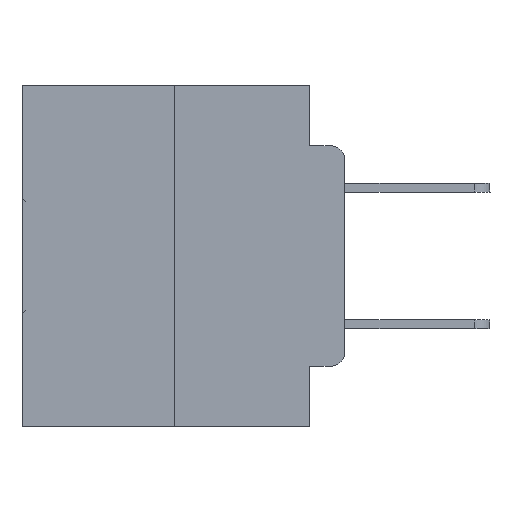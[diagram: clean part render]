
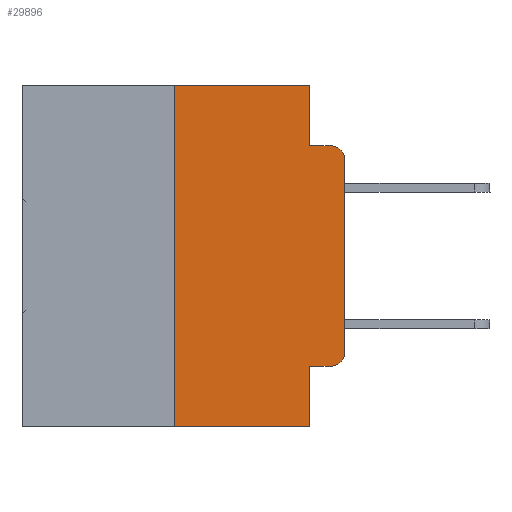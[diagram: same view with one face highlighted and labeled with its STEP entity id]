
A CAD part, left-side view. The second image highlights one B-rep face of the part: STEP entity #29896.
In plain terms, the highlighted planar face has unit normal (-1, 0, 0).
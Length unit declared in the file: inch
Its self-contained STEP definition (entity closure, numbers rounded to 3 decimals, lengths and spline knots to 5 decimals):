
#251 = CARTESIAN_POINT ( 'NONE',  ( 0., 0.051, 0. ) ) ;
#461 = DIRECTION ( 'NONE',  ( 0., -1., 0. ) ) ;
#693 = DIRECTION ( 'NONE',  ( 0., 0., -1. ) ) ;
#1425 = VERTEX_POINT ( 'NONE', #11862 ) ;
#2590 = EDGE_CURVE ( 'NONE', #15403, #14087, #17439, .T. ) ;
#2677 = CARTESIAN_POINT ( 'NONE',  ( 0., 0.02, -0.0885 ) ) ;
#3203 = ORIENTED_EDGE ( 'NONE', *, *, #27578, .F. ) ;
#3482 = DIRECTION ( 'NONE',  ( 0., 0., -1. ) ) ;
#4681 = VECTOR ( 'NONE', #26832, 39.37008 ) ;
#4895 = ORIENTED_EDGE ( 'NONE', *, *, #20392, .T. ) ;
#5065 = VERTEX_POINT ( 'NONE', #13213 ) ;
#5079 = DIRECTION ( 'NONE',  ( -1., 0., 0. ) ) ;
#5665 = VECTOR ( 'NONE', #3482, 39.37008 ) ;
#5751 = CARTESIAN_POINT ( 'NONE',  ( 0., 0.051, -0.0885 ) ) ;
#7278 = EDGE_LOOP ( 'NONE', ( #19356, #32221, #27147, #3203, #12498, #8711, #18273, #20991, #24960, #4895 ) ) ;
#7427 = CARTESIAN_POINT ( 'NONE',  ( 0., 0.051, -0.4115 ) ) ;
#7637 = DIRECTION ( 'NONE',  ( 0., 0., -1. ) ) ;
#8510 = DIRECTION ( 'NONE',  ( 0., -1., 0. ) ) ;
#8711 = ORIENTED_EDGE ( 'NONE', *, *, #25405, .F. ) ;
#9150 = EDGE_CURVE ( 'NONE', #17192, #9315, #14509, .T. ) ;
#9315 = VERTEX_POINT ( 'NONE', #21092 ) ;
#10028 = CARTESIAN_POINT ( 'NONE',  ( 0., 0.02, -0.3915 ) ) ;
#10071 = CARTESIAN_POINT ( 'NONE',  ( 0., 0., 0. ) ) ;
#10776 = EDGE_CURVE ( 'NONE', #25281, #31909, #28466, .T. ) ;
#11602 = DIRECTION ( 'NONE',  ( 0., -1., 0. ) ) ;
#11862 = CARTESIAN_POINT ( 'NONE',  ( 0., 0., -0.3915 ) ) ;
#11918 = AXIS2_PLACEMENT_3D ( 'NONE', #22480, #22384, #7637 ) ;
#12401 = LINE ( 'NONE', #10071, #26482 ) ;
#12488 = PLANE ( 'NONE',  #11918 ) ;
#12498 = ORIENTED_EDGE ( 'NONE', *, *, #10776, .F. ) ;
#12736 = LINE ( 'NONE', #16044, #5665 ) ;
#13051 = CARTESIAN_POINT ( 'NONE',  ( 0., 0.02, -0.1085 ) ) ;
#13213 = CARTESIAN_POINT ( 'NONE',  ( 0., 0.051, -0.5 ) ) ;
#14087 = VERTEX_POINT ( 'NONE', #2677 ) ;
#14341 = CARTESIAN_POINT ( 'NONE',  ( 0., 0.473, 0. ) ) ;
#14509 = LINE ( 'NONE', #7427, #31758 ) ;
#15403 = VERTEX_POINT ( 'NONE', #30290 ) ;
#16044 = CARTESIAN_POINT ( 'NONE',  ( 0., 0.051, 0. ) ) ;
#16433 = CARTESIAN_POINT ( 'NONE',  ( 0., 0.25, 0. ) ) ;
#17080 = CARTESIAN_POINT ( 'NONE',  ( 0., 0.051, 0. ) ) ;
#17192 = VERTEX_POINT ( 'NONE', #25063 ) ;
#17289 = EDGE_CURVE ( 'NONE', #29818, #14087, #26398, .T. ) ;
#17439 = LINE ( 'NONE', #5751, #18234 ) ;
#17487 = DIRECTION ( 'NONE',  ( 0., -1., 0. ) ) ;
#17661 = VERTEX_POINT ( 'NONE', #20322 ) ;
#18234 = VECTOR ( 'NONE', #461, 39.37008 ) ;
#18273 = ORIENTED_EDGE ( 'NONE', *, *, #30205, .T. ) ;
#19356 = ORIENTED_EDGE ( 'NONE', *, *, #21573, .T. ) ;
#20322 = CARTESIAN_POINT ( 'NONE',  ( 0., 0.25, -0.5 ) ) ;
#20392 = EDGE_CURVE ( 'NONE', #9315, #1425, #24549, .T. ) ;
#20574 = VECTOR ( 'NONE', #32305, 39.37008 ) ;
#20762 = DIRECTION ( 'NONE',  ( -1., 0., 0. ) ) ;
#20991 = ORIENTED_EDGE ( 'NONE', *, *, #28213, .F. ) ;
#21092 = CARTESIAN_POINT ( 'NONE',  ( 0., 0.02, -0.4115 ) ) ;
#21524 = AXIS2_PLACEMENT_3D ( 'NONE', #10028, #5079, #30175 ) ;
#21573 = EDGE_CURVE ( 'NONE', #1425, #29818, #12401, .T. ) ;
#22082 = AXIS2_PLACEMENT_3D ( 'NONE', #13051, #20762, #693 ) ;
#22384 = DIRECTION ( 'NONE',  ( 1., 0., 0. ) ) ;
#22480 = CARTESIAN_POINT ( 'NONE',  ( 0., 0.473, 0. ) ) ;
#22522 = LINE ( 'NONE', #17080, #20574 ) ;
#23540 = VECTOR ( 'NONE', #8510, 39.37008 ) ;
#23568 = CARTESIAN_POINT ( 'NONE',  ( 0., 0.473, -0.5 ) ) ;
#24520 = CARTESIAN_POINT ( 'NONE',  ( 0., 0.25, 0. ) ) ;
#24549 = CIRCLE ( 'NONE', #21524, 0.02 ) ;
#24636 = LINE ( 'NONE', #24520, #4681 ) ;
#24934 = VECTOR ( 'NONE', #11602, 39.37008 ) ;
#24960 = ORIENTED_EDGE ( 'NONE', *, *, #9150, .T. ) ;
#25063 = CARTESIAN_POINT ( 'NONE',  ( 0., 0.051, -0.4115 ) ) ;
#25281 = VERTEX_POINT ( 'NONE', #16433 ) ;
#25405 = EDGE_CURVE ( 'NONE', #17661, #25281, #24636, .T. ) ;
#25519 = LINE ( 'NONE', #23568, #23540 ) ;
#26398 = CIRCLE ( 'NONE', #22082, 0.02 ) ;
#26482 = VECTOR ( 'NONE', #27236, 39.37008 ) ;
#26832 = DIRECTION ( 'NONE',  ( 0., 0., 1. ) ) ;
#27147 = ORIENTED_EDGE ( 'NONE', *, *, #2590, .F. ) ;
#27236 = DIRECTION ( 'NONE',  ( 0., 0., 1. ) ) ;
#27578 = EDGE_CURVE ( 'NONE', #31909, #15403, #22522, .T. ) ;
#28213 = EDGE_CURVE ( 'NONE', #17192, #5065, #12736, .T. ) ;
#28466 = LINE ( 'NONE', #14341, #24934 ) ;
#29790 = CARTESIAN_POINT ( 'NONE',  ( 0., 0., -0.1085 ) ) ;
#29818 = VERTEX_POINT ( 'NONE', #29790 ) ;
#29896 = ADVANCED_FACE ( 'NONE', ( #32233 ), #12488, .F. ) ;
#30175 = DIRECTION ( 'NONE',  ( 0., 0., -1. ) ) ;
#30205 = EDGE_CURVE ( 'NONE', #17661, #5065, #25519, .T. ) ;
#30290 = CARTESIAN_POINT ( 'NONE',  ( 0., 0.051, -0.0885 ) ) ;
#31758 = VECTOR ( 'NONE', #17487, 39.37008 ) ;
#31909 = VERTEX_POINT ( 'NONE', #251 ) ;
#32221 = ORIENTED_EDGE ( 'NONE', *, *, #17289, .T. ) ;
#32233 = FACE_OUTER_BOUND ( 'NONE', #7278, .T. ) ;
#32305 = DIRECTION ( 'NONE',  ( 0., 0., -1. ) ) ;
